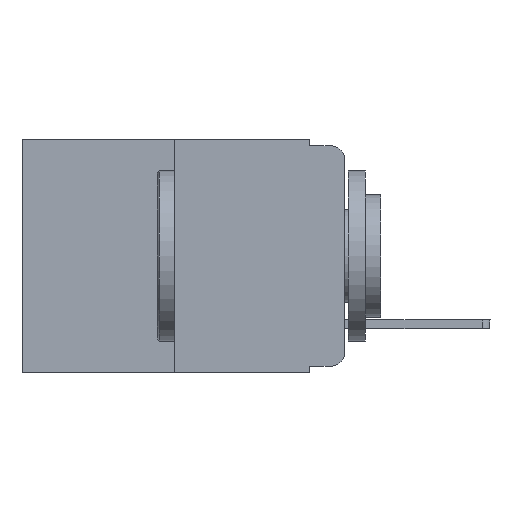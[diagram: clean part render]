
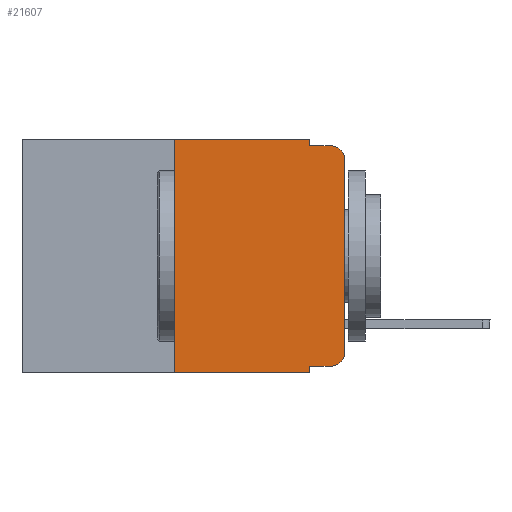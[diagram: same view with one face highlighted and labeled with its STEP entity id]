
A CAD part, left-side view. The second image highlights one B-rep face of the part: STEP entity #21607.
In plain terms, the highlighted planar face has unit normal (-1, 0, 0).
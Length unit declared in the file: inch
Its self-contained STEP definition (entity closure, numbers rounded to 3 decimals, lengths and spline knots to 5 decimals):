
#61 = EDGE_CURVE ( 'NONE', #6216, #3515, #13673, .T. ) ;
#317 = ORIENTED_EDGE ( 'NONE', *, *, #5452, .F. ) ;
#1232 = ORIENTED_EDGE ( 'NONE', *, *, #5340, .F. ) ;
#1444 = CARTESIAN_POINT ( 'NONE',  ( 0., 0.051, 0. ) ) ;
#1512 = DIRECTION ( 'NONE',  ( 0., 0., -1. ) ) ;
#1755 = CARTESIAN_POINT ( 'NONE',  ( 0., 0.02, -0.01 ) ) ;
#1798 = CARTESIAN_POINT ( 'NONE',  ( 0., 0.02, -0.03 ) ) ;
#1869 = LINE ( 'NONE', #3957, #12546 ) ;
#1981 = VECTOR ( 'NONE', #12377, 39.37008 ) ;
#2081 = ORIENTED_EDGE ( 'NONE', *, *, #17916, .T. ) ;
#2167 = CIRCLE ( 'NONE', #18950, 0.02 ) ;
#2206 = EDGE_CURVE ( 'NONE', #3515, #11620, #1869, .T. ) ;
#2338 = CIRCLE ( 'NONE', #16145, 0.02 ) ;
#2958 = VERTEX_POINT ( 'NONE', #4592 ) ;
#3515 = VERTEX_POINT ( 'NONE', #1444 ) ;
#3957 = CARTESIAN_POINT ( 'NONE',  ( 0., 0.051, 0. ) ) ;
#3997 = VECTOR ( 'NONE', #18525, 39.37008 ) ;
#4372 = CARTESIAN_POINT ( 'NONE',  ( 0., 0.473, -0.343 ) ) ;
#4457 = DIRECTION ( 'NONE',  ( 1., 0., 0. ) ) ;
#4474 = DIRECTION ( 'NONE',  ( 0., 0., 1. ) ) ;
#4592 = CARTESIAN_POINT ( 'NONE',  ( 0., 0., -0.313 ) ) ;
#5340 = EDGE_CURVE ( 'NONE', #11620, #7750, #11030, .T. ) ;
#5452 = EDGE_CURVE ( 'NONE', #14155, #6216, #17343, .T. ) ;
#5648 = CARTESIAN_POINT ( 'NONE',  ( 0., 0.02, -0.333 ) ) ;
#5760 = DIRECTION ( 'NONE',  ( 0., -1., 0. ) ) ;
#6062 = CARTESIAN_POINT ( 'NONE',  ( 0., 0.051, -0.333 ) ) ;
#6216 = VERTEX_POINT ( 'NONE', #11184 ) ;
#6641 = EDGE_CURVE ( 'NONE', #14155, #17482, #16752, .T. ) ;
#6922 = VECTOR ( 'NONE', #4474, 39.37008 ) ;
#7015 = EDGE_CURVE ( 'NONE', #13433, #2958, #2167, .T. ) ;
#7127 = DIRECTION ( 'NONE',  ( 0., 0., -1. ) ) ;
#7750 = VERTEX_POINT ( 'NONE', #1755 ) ;
#8860 = EDGE_LOOP ( 'NONE', ( #12499, #2081, #1232, #20254, #15503, #317, #19028, #13430, #19924, #10290 ) ) ;
#9046 = DIRECTION ( 'NONE',  ( 0., 0., 1. ) ) ;
#9109 = DIRECTION ( 'NONE',  ( -1., 0., 0. ) ) ;
#9441 = VECTOR ( 'NONE', #1512, 39.37008 ) ;
#10290 = ORIENTED_EDGE ( 'NONE', *, *, #7015, .T. ) ;
#10501 = EDGE_CURVE ( 'NONE', #22016, #17482, #14000, .T. ) ;
#11030 = LINE ( 'NONE', #14661, #18885 ) ;
#11184 = CARTESIAN_POINT ( 'NONE',  ( 0., 0.25, 0. ) ) ;
#11620 = VERTEX_POINT ( 'NONE', #20346 ) ;
#12124 = CARTESIAN_POINT ( 'NONE',  ( 0., 0.051, 0. ) ) ;
#12377 = DIRECTION ( 'NONE',  ( 0., -1., 0. ) ) ;
#12499 = ORIENTED_EDGE ( 'NONE', *, *, #15936, .T. ) ;
#12546 = VECTOR ( 'NONE', #15994, 39.37008 ) ;
#13140 = VECTOR ( 'NONE', #9046, 39.37008 ) ;
#13208 = CARTESIAN_POINT ( 'NONE',  ( 0., 0.473, 0. ) ) ;
#13355 = FACE_OUTER_BOUND ( 'NONE', #8860, .T. ) ;
#13430 = ORIENTED_EDGE ( 'NONE', *, *, #10501, .F. ) ;
#13433 = VERTEX_POINT ( 'NONE', #5648 ) ;
#13673 = LINE ( 'NONE', #13208, #22533 ) ;
#14000 = LINE ( 'NONE', #12124, #9441 ) ;
#14155 = VERTEX_POINT ( 'NONE', #15875 ) ;
#14248 = LINE ( 'NONE', #19637, #1981 ) ;
#14306 = CARTESIAN_POINT ( 'NONE',  ( 0., 0.051, -0.343 ) ) ;
#14629 = DIRECTION ( 'NONE',  ( 0., 0., -1. ) ) ;
#14661 = CARTESIAN_POINT ( 'NONE',  ( 0., 0.051, -0.01 ) ) ;
#15189 = CARTESIAN_POINT ( 'NONE',  ( 0., 0., -0.03 ) ) ;
#15196 = DIRECTION ( 'NONE',  ( 0., -1., 0. ) ) ;
#15503 = ORIENTED_EDGE ( 'NONE', *, *, #61, .F. ) ;
#15875 = CARTESIAN_POINT ( 'NONE',  ( 0., 0.25, -0.343 ) ) ;
#15936 = EDGE_CURVE ( 'NONE', #2958, #16854, #21695, .T. ) ;
#15994 = DIRECTION ( 'NONE',  ( 0., 0., -1. ) ) ;
#16145 = AXIS2_PLACEMENT_3D ( 'NONE', #1798, #9109, #7127 ) ;
#16752 = LINE ( 'NONE', #4372, #3997 ) ;
#16854 = VERTEX_POINT ( 'NONE', #15189 ) ;
#17104 = CARTESIAN_POINT ( 'NONE',  ( 0., 0.25, 0. ) ) ;
#17343 = LINE ( 'NONE', #17104, #6922 ) ;
#17482 = VERTEX_POINT ( 'NONE', #14306 ) ;
#17916 = EDGE_CURVE ( 'NONE', #16854, #7750, #2338, .T. ) ;
#18367 = DIRECTION ( 'NONE',  ( -1., 0., 0. ) ) ;
#18525 = DIRECTION ( 'NONE',  ( 0., -1., 0. ) ) ;
#18841 = DIRECTION ( 'NONE',  ( 0., 0., -1. ) ) ;
#18885 = VECTOR ( 'NONE', #5760, 39.37008 ) ;
#18950 = AXIS2_PLACEMENT_3D ( 'NONE', #21890, #18367, #14629 ) ;
#19028 = ORIENTED_EDGE ( 'NONE', *, *, #6641, .T. ) ;
#19637 = CARTESIAN_POINT ( 'NONE',  ( 0., 0.051, -0.333 ) ) ;
#19676 = EDGE_CURVE ( 'NONE', #22016, #13433, #14248, .T. ) ;
#19924 = ORIENTED_EDGE ( 'NONE', *, *, #19676, .T. ) ;
#19945 = CARTESIAN_POINT ( 'NONE',  ( 0., 0., 0. ) ) ;
#20247 = PLANE ( 'NONE',  #21071 ) ;
#20254 = ORIENTED_EDGE ( 'NONE', *, *, #2206, .F. ) ;
#20346 = CARTESIAN_POINT ( 'NONE',  ( 0., 0.051, -0.01 ) ) ;
#21071 = AXIS2_PLACEMENT_3D ( 'NONE', #22354, #4457, #18841 ) ;
#21607 = ADVANCED_FACE ( 'NONE', ( #13355 ), #20247, .F. ) ;
#21695 = LINE ( 'NONE', #19945, #13140 ) ;
#21890 = CARTESIAN_POINT ( 'NONE',  ( 0., 0.02, -0.313 ) ) ;
#22016 = VERTEX_POINT ( 'NONE', #6062 ) ;
#22354 = CARTESIAN_POINT ( 'NONE',  ( 0., 0.473, 0. ) ) ;
#22533 = VECTOR ( 'NONE', #15196, 39.37008 ) ;
